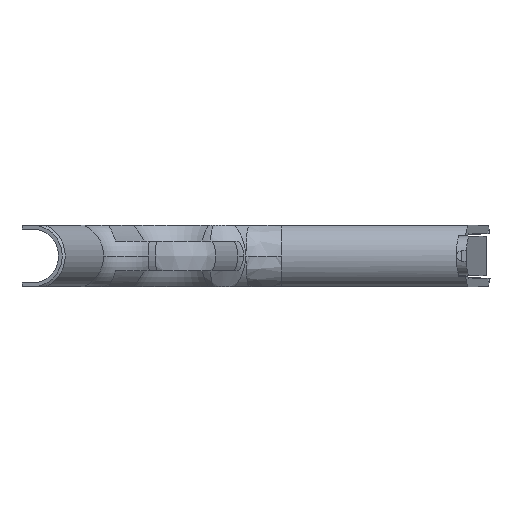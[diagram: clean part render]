
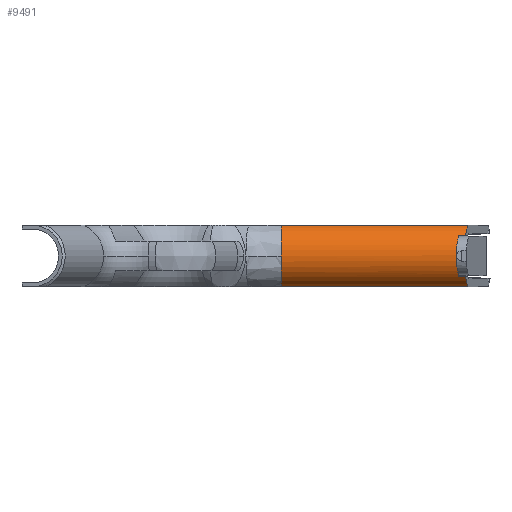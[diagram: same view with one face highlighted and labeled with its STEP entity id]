
A CAD part, left-side view. The second image highlights one B-rep face of the part: STEP entity #9491.
In plain terms, the highlighted cylindrical face has radius 10.319 mm (diameter 20.638 mm), a partial arc.
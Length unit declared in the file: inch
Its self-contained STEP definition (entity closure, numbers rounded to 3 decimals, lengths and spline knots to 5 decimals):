
#5115=CARTESIAN_POINT('',(0.376,-1.75645,-1.65206));
#5116=VERTEX_POINT('',#5115);
#5124=CARTESIAN_POINT('',(0.376,-3.94251,-2.34132));
#5125=VERTEX_POINT('',#5124);
#5126=CARTESIAN_POINT('',(0.376,-3.94251,-2.34132));
#5127=DIRECTION('',(0.0,0.954,0.301));
#5128=VECTOR('',#5127,2.29215);
#5129=LINE('',#5126,#5128);
#5130=EDGE_CURVE('',#5125,#5116,#5129,.T.);
#5458=CARTESIAN_POINT('',(0.254,-3.96666,-2.17779));
#5459=VERTEX_POINT('',#5458);
#5460=CARTESIAN_POINT('',(-0.00001,-3.91975,-2.49545));
#5461=DIRECTION('',(0.,-0.989,-0.146));
#5462=DIRECTION('',(-0.001,0.146,-0.989));
#5463=AXIS2_PLACEMENT_3D('',#5460,#5461,#5462);
#5464=ELLIPSE('',#5463,0.41144,0.40626);
#5465=EDGE_CURVE('',#5125,#5459,#5464,.T.);
#7790=CARTESIAN_POINT('',(0.254,-3.88456,-2.1519));
#7791=VERTEX_POINT('',#7790);
#7792=CARTESIAN_POINT('',(0.254,-3.96666,-2.17779));
#7793=DIRECTION('',(0.,0.954,0.301));
#7794=VECTOR('',#7793,0.08608);
#7795=LINE('',#7792,#7794);
#7796=EDGE_CURVE('',#5459,#7791,#7795,.T.);
#7815=CARTESIAN_POINT('',(-0.254,-3.88456,-2.1519));
#7816=VERTEX_POINT('',#7815);
#7817=CARTESIAN_POINT('',(0.,-3.83765,-2.46955));
#7818=DIRECTION('',(0.,-0.989,-0.146));
#7819=DIRECTION('',(0.,0.146,-0.989));
#7820=AXIS2_PLACEMENT_3D('',#7817,#7818,#7819);
#7821=ELLIPSE('',#7820,0.41143,0.40625);
#7822=EDGE_CURVE('',#7791,#7816,#7821,.T.);
#7839=CARTESIAN_POINT('',(-0.254,-3.96666,-2.17779));
#7840=VERTEX_POINT('',#7839);
#7841=CARTESIAN_POINT('',(-0.254,-3.88456,-2.1519));
#7842=DIRECTION('',(0.,-0.954,-0.301));
#7843=VECTOR('',#7842,0.08608);
#7844=LINE('',#7841,#7843);
#7845=EDGE_CURVE('',#7816,#7840,#7844,.T.);
#7904=CARTESIAN_POINT('',(-0.376,-1.75645,-1.65206));
#7905=VERTEX_POINT('',#7904);
#7915=CARTESIAN_POINT('',(0.,-1.83235,-1.41132));
#7916=VERTEX_POINT('',#7915);
#7917=CARTESIAN_POINT('',(0.0,-1.71019,-1.79877));
#7918=DIRECTION('',(0.0,0.954,0.301));
#7919=DIRECTION('',(0.0,0.301,-0.954));
#7920=AXIS2_PLACEMENT_3D('',#7917,#7918,#7919);
#7921=CIRCLE('',#7920,0.40625);
#7922=EDGE_CURVE('',#7905,#7916,#7921,.T.);
#8262=CARTESIAN_POINT('',(-0.376,-3.94251,-2.34132));
#8263=VERTEX_POINT('',#8262);
#8270=CARTESIAN_POINT('',(-0.376,-3.94251,-2.34132));
#8271=DIRECTION('',(0.,0.954,0.301));
#8272=VECTOR('',#8271,2.29215);
#8273=LINE('',#8270,#8272);
#8274=EDGE_CURVE('',#8263,#7905,#8273,.T.);
#9434=CARTESIAN_POINT('',(0.00001,-3.91975,-2.49545));
#9435=DIRECTION('',(0.,-0.989,-0.146));
#9436=DIRECTION('',(0.001,0.146,-0.989));
#9437=AXIS2_PLACEMENT_3D('',#9434,#9435,#9436);
#9438=ELLIPSE('',#9437,0.41144,0.40626);
#9439=EDGE_CURVE('',#7840,#8263,#9438,.T.);
#9469=CARTESIAN_POINT('',(0.0,-1.71019,-1.79877));
#9470=DIRECTION('',(0.0,-0.954,-0.301));
#9471=DIRECTION('',(0.0,0.301,-0.954));
#9472=AXIS2_PLACEMENT_3D('',#9469,#9470,#9471);
#9473=CYLINDRICAL_SURFACE('',#9472,0.40625);
#9474=ORIENTED_EDGE('',*,*,#7822,.F.);
#9475=ORIENTED_EDGE('',*,*,#7796,.F.);
#9476=ORIENTED_EDGE('',*,*,#5465,.F.);
#9477=ORIENTED_EDGE('',*,*,#5130,.T.);
#9478=CARTESIAN_POINT('',(0.,-1.71019,-1.79877));
#9479=DIRECTION('',(0.,0.954,0.301));
#9480=DIRECTION('',(0.926,-0.114,0.361));
#9481=AXIS2_PLACEMENT_3D('',#9478,#9479,#9480);
#9482=CIRCLE('',#9481,0.40625);
#9483=EDGE_CURVE('',#7916,#5116,#9482,.T.);
#9484=ORIENTED_EDGE('',*,*,#9483,.F.);
#9485=ORIENTED_EDGE('',*,*,#7922,.F.);
#9486=ORIENTED_EDGE('',*,*,#8274,.F.);
#9487=ORIENTED_EDGE('',*,*,#9439,.F.);
#9488=ORIENTED_EDGE('',*,*,#7845,.F.);
#9489=EDGE_LOOP('',(#9474,#9475,#9476,#9477,#9484,#9485,#9486,#9487,#9488));
#9490=FACE_OUTER_BOUND('',#9489,.T.);
#9491=ADVANCED_FACE('',(#9490),#9473,.T.);
